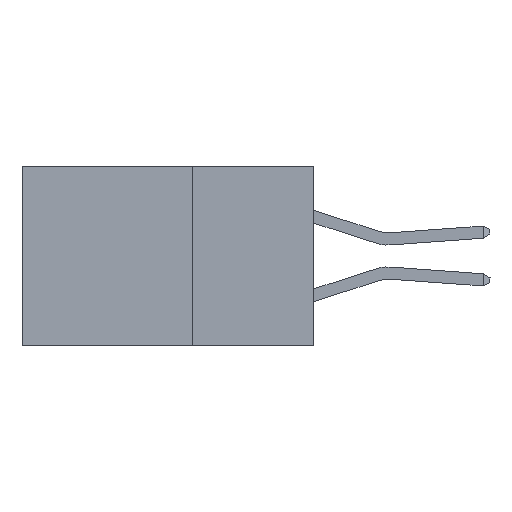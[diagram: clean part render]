
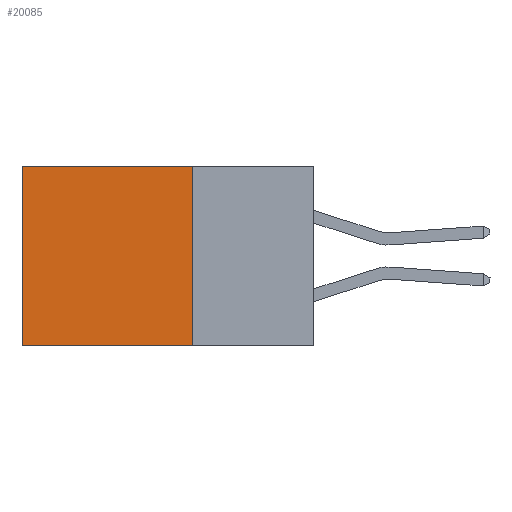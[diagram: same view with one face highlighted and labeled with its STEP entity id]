
A CAD part, left-side view. The second image highlights one B-rep face of the part: STEP entity #20085.
In plain terms, the highlighted planar face has unit normal (-1, 0, 0).
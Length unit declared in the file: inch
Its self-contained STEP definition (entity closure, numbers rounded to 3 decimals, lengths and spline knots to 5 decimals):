
#123 = VECTOR ( 'NONE', #15360, 39.37008 ) ;
#168 = CARTESIAN_POINT ( 'NONE',  ( 0.2875, 0.6, 0. ) ) ;
#917 = DIRECTION ( 'NONE',  ( 1., 0., 0. ) ) ;
#1127 = LINE ( 'NONE', #8455, #16733 ) ;
#1985 = VECTOR ( 'NONE', #8845, 39.37008 ) ;
#3391 = VERTEX_POINT ( 'NONE', #14969 ) ;
#4881 = PLANE ( 'NONE',  #6916 ) ;
#5523 = EDGE_LOOP ( 'NONE', ( #14320, #8966, #10417, #24940 ) ) ;
#5754 = EDGE_CURVE ( 'NONE', #11892, #3391, #25218, .T. ) ;
#6486 = CARTESIAN_POINT ( 'NONE',  ( 0.2875, 0.25, -0.37 ) ) ;
#6558 = FACE_OUTER_BOUND ( 'NONE', #5523, .T. ) ;
#6916 = AXIS2_PLACEMENT_3D ( 'NONE', #10547, #917, #18885 ) ;
#7895 = CARTESIAN_POINT ( 'NONE',  ( 0.2875, 0.25, -0.37 ) ) ;
#8455 = CARTESIAN_POINT ( 'NONE',  ( 0.2875, 0.25, 0. ) ) ;
#8845 = DIRECTION ( 'NONE',  ( 0., 1., 0. ) ) ;
#8966 = ORIENTED_EDGE ( 'NONE', *, *, #18694, .F. ) ;
#10417 = ORIENTED_EDGE ( 'NONE', *, *, #24934, .F. ) ;
#10470 = CARTESIAN_POINT ( 'NONE',  ( 0.2875, 0.6, 0. ) ) ;
#10547 = CARTESIAN_POINT ( 'NONE',  ( 0.2875, 0.25, 0. ) ) ;
#11055 = VECTOR ( 'NONE', #11983, 39.37008 ) ;
#11892 = VERTEX_POINT ( 'NONE', #10470 ) ;
#11983 = DIRECTION ( 'NONE',  ( 0., 0., -1. ) ) ;
#13236 = EDGE_CURVE ( 'NONE', #16360, #11892, #1127, .T. ) ;
#14128 = LINE ( 'NONE', #25061, #123 ) ;
#14320 = ORIENTED_EDGE ( 'NONE', *, *, #5754, .T. ) ;
#14969 = CARTESIAN_POINT ( 'NONE',  ( 0.2875, 0.6, -0.37 ) ) ;
#15348 = VERTEX_POINT ( 'NONE', #7895 ) ;
#15360 = DIRECTION ( 'NONE',  ( 0., 0., -1. ) ) ;
#16031 = LINE ( 'NONE', #6486, #1985 ) ;
#16360 = VERTEX_POINT ( 'NONE', #20834 ) ;
#16733 = VECTOR ( 'NONE', #20457, 39.37008 ) ;
#18694 = EDGE_CURVE ( 'NONE', #15348, #3391, #16031, .T. ) ;
#18885 = DIRECTION ( 'NONE',  ( 0., 0., -1. ) ) ;
#20085 = ADVANCED_FACE ( 'NONE', ( #6558 ), #4881, .F. ) ;
#20457 = DIRECTION ( 'NONE',  ( 0., 1., 0. ) ) ;
#20834 = CARTESIAN_POINT ( 'NONE',  ( 0.2875, 0.25, 0. ) ) ;
#24934 = EDGE_CURVE ( 'NONE', #16360, #15348, #14128, .T. ) ;
#24940 = ORIENTED_EDGE ( 'NONE', *, *, #13236, .T. ) ;
#25061 = CARTESIAN_POINT ( 'NONE',  ( 0.2875, 0.25, 0. ) ) ;
#25218 = LINE ( 'NONE', #168, #11055 ) ;
